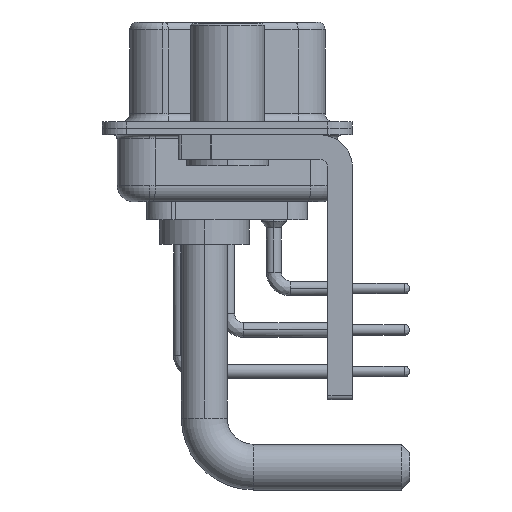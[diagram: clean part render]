
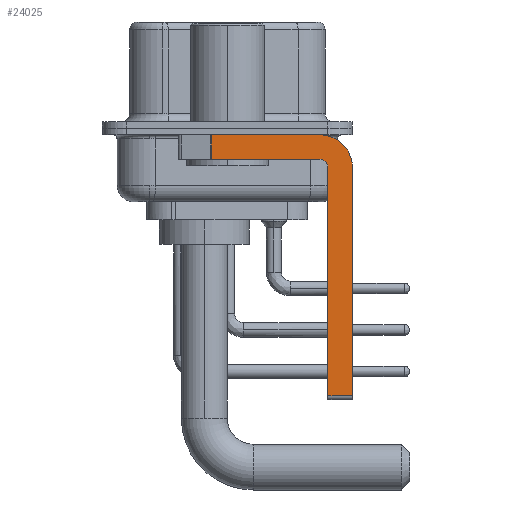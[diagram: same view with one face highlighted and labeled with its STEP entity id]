
A CAD part, left-side view. The second image highlights one B-rep face of the part: STEP entity #24025.
In plain terms, the highlighted planar face has unit normal (-1, 0, 0).
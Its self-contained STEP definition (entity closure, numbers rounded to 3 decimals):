
#215 = VECTOR ( 'NONE', #29431, 1000. ) ;
#626 = CARTESIAN_POINT ( 'NONE',  ( -2.9, 0.978, -1.9 ) ) ;
#648 = CARTESIAN_POINT ( 'NONE',  ( -2.9, -5.65, -16.35 ) ) ;
#710 = ORIENTED_EDGE ( 'NONE', *, *, #27402, .T. ) ;
#1178 = VECTOR ( 'NONE', #26431, 1000. ) ;
#1651 = EDGE_CURVE ( 'NONE', #28791, #3638, #14726, .T. ) ;
#2464 = CARTESIAN_POINT ( 'NONE',  ( -2.9, -5.65, -1.9 ) ) ;
#2651 = ORIENTED_EDGE ( 'NONE', *, *, #33566, .F. ) ;
#2950 = DIRECTION ( 'NONE',  ( 0., 0., 1. ) ) ;
#2990 = AXIS2_PLACEMENT_3D ( 'NONE', #17656, #20810, #23417 ) ;
#3638 = VERTEX_POINT ( 'NONE', #19497 ) ;
#3813 = EDGE_CURVE ( 'NONE', #23371, #3638, #24058, .T. ) ;
#4283 = VECTOR ( 'NONE', #29276, 1000. ) ;
#5415 = ORIENTED_EDGE ( 'NONE', *, *, #33818, .F. ) ;
#5670 = AXIS2_PLACEMENT_3D ( 'NONE', #7630, #13008, #27304 ) ;
#5735 = LINE ( 'NONE', #31746, #23673 ) ;
#6757 = LINE ( 'NONE', #32041, #27175 ) ;
#7630 = CARTESIAN_POINT ( 'NONE',  ( -2.9, -5.65, -2.4 ) ) ;
#9410 = VECTOR ( 'NONE', #23598, 1000. ) ;
#10102 = CARTESIAN_POINT ( 'NONE',  ( -2.9, -5.65, -0.4 ) ) ;
#11384 = EDGE_LOOP ( 'NONE', ( #31639, #27681, #15989, #20294, #5415, #710, #2651, #30040 ) ) ;
#12195 = DIRECTION ( 'NONE',  ( 0., 0., -1. ) ) ;
#12492 = VERTEX_POINT ( 'NONE', #26477 ) ;
#13008 = DIRECTION ( 'NONE',  ( -1., 0., 0. ) ) ;
#13148 = CIRCLE ( 'NONE', #2990, 2. ) ;
#14726 = LINE ( 'NONE', #626, #1178 ) ;
#14783 = CARTESIAN_POINT ( 'NONE',  ( -2.9, -5.65, -2.4 ) ) ;
#15303 = VERTEX_POINT ( 'NONE', #32278 ) ;
#15989 = ORIENTED_EDGE ( 'NONE', *, *, #3813, .F. ) ;
#17656 = CARTESIAN_POINT ( 'NONE',  ( -2.9, -5.65, -2.4 ) ) ;
#19040 = VERTEX_POINT ( 'NONE', #24506 ) ;
#19497 = CARTESIAN_POINT ( 'NONE',  ( -2.9, 0.978, -1.9 ) ) ;
#20294 = ORIENTED_EDGE ( 'NONE', *, *, #21965, .F. ) ;
#20810 = DIRECTION ( 'NONE',  ( 1., 0., 0. ) ) ;
#21459 = CARTESIAN_POINT ( 'NONE',  ( -2.9, -5.65, -1.9 ) ) ;
#21965 = EDGE_CURVE ( 'NONE', #15303, #23371, #26425, .T. ) ;
#22793 = DIRECTION ( 'NONE',  ( 1., 0., 0. ) ) ;
#22973 = PLANE ( 'NONE',  #33692 ) ;
#23371 = VERTEX_POINT ( 'NONE', #2464 ) ;
#23417 = DIRECTION ( 'NONE',  ( 0., 0., -1. ) ) ;
#23522 = FACE_OUTER_BOUND ( 'NONE', #11384, .T. ) ;
#23598 = DIRECTION ( 'NONE',  ( 0., 0., -1. ) ) ;
#23673 = VECTOR ( 'NONE', #2950, 1000. ) ;
#24025 = ADVANCED_FACE ( 'NONE', ( #23522 ), #22973, .F. ) ;
#24058 = LINE ( 'NONE', #21459, #4283 ) ;
#24476 = EDGE_CURVE ( 'NONE', #28791, #32511, #6757, .T. ) ;
#24506 = CARTESIAN_POINT ( 'NONE',  ( -2.9, -6.15, -16.35 ) ) ;
#26425 = CIRCLE ( 'NONE', #5670, 0.5 ) ;
#26431 = DIRECTION ( 'NONE',  ( 0., 0., -1. ) ) ;
#26477 = CARTESIAN_POINT ( 'NONE',  ( -2.9, -7.65, -2.4 ) ) ;
#27064 = CARTESIAN_POINT ( 'NONE',  ( -2.9, -7.65, -16.35 ) ) ;
#27175 = VECTOR ( 'NONE', #32396, 1000. ) ;
#27293 = LINE ( 'NONE', #35124, #9410 ) ;
#27304 = DIRECTION ( 'NONE',  ( 0., 0., 1. ) ) ;
#27402 = EDGE_CURVE ( 'NONE', #19040, #34026, #34657, .T. ) ;
#27681 = ORIENTED_EDGE ( 'NONE', *, *, #1651, .T. ) ;
#28791 = VERTEX_POINT ( 'NONE', #32239 ) ;
#29276 = DIRECTION ( 'NONE',  ( 0., 1., 0. ) ) ;
#29431 = DIRECTION ( 'NONE',  ( 0., -1., 0. ) ) ;
#30040 = ORIENTED_EDGE ( 'NONE', *, *, #36734, .F. ) ;
#31639 = ORIENTED_EDGE ( 'NONE', *, *, #24476, .F. ) ;
#31746 = CARTESIAN_POINT ( 'NONE',  ( -2.9, -6.15, -16.6 ) ) ;
#32041 = CARTESIAN_POINT ( 'NONE',  ( -2.9, 3., -0.4 ) ) ;
#32239 = CARTESIAN_POINT ( 'NONE',  ( -2.9, 0.978, -0.4 ) ) ;
#32278 = CARTESIAN_POINT ( 'NONE',  ( -2.9, -6.15, -2.4 ) ) ;
#32396 = DIRECTION ( 'NONE',  ( 0., -1., 0. ) ) ;
#32511 = VERTEX_POINT ( 'NONE', #10102 ) ;
#33566 = EDGE_CURVE ( 'NONE', #12492, #34026, #27293, .T. ) ;
#33692 = AXIS2_PLACEMENT_3D ( 'NONE', #14783, #22793, #12195 ) ;
#33818 = EDGE_CURVE ( 'NONE', #19040, #15303, #5735, .T. ) ;
#34026 = VERTEX_POINT ( 'NONE', #27064 ) ;
#34657 = LINE ( 'NONE', #648, #215 ) ;
#35124 = CARTESIAN_POINT ( 'NONE',  ( -2.9, -7.65, -2.4 ) ) ;
#36734 = EDGE_CURVE ( 'NONE', #32511, #12492, #13148, .T. ) ;
